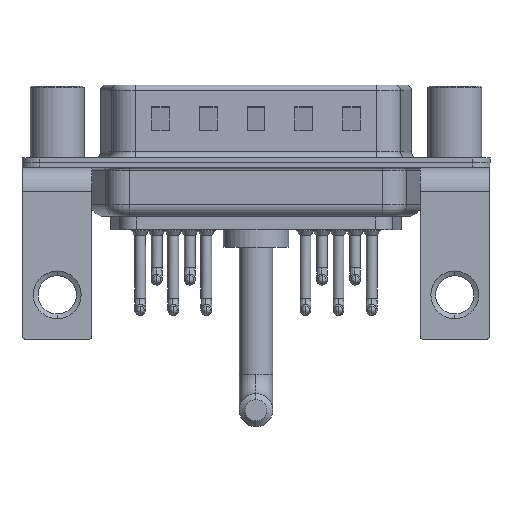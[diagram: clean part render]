
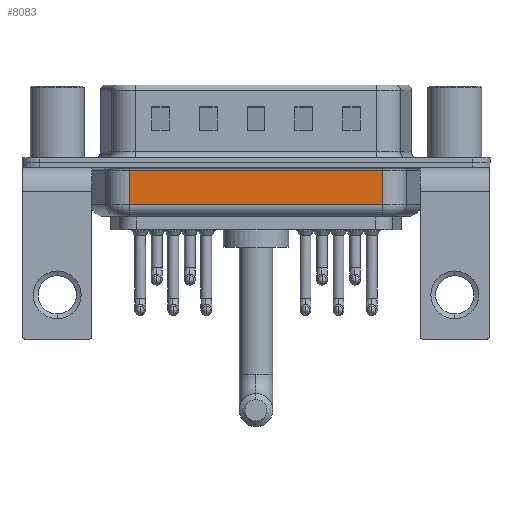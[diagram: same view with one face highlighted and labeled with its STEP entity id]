
A CAD part, front view. The second image highlights one B-rep face of the part: STEP entity #8083.
In plain terms, the highlighted planar face has unit normal (0, -1, 0).
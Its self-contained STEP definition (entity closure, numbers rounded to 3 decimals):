
#132 = CARTESIAN_POINT ( 'NONE',  ( 27.269, -5.35, -0.65 ) ) ;
#487 = CARTESIAN_POINT ( 'NONE',  ( 6.031, -5.35, -0.65 ) ) ;
#1815 = ORIENTED_EDGE ( 'NONE', *, *, #18002, .T. ) ;
#2347 = VECTOR ( 'NONE', #18919, 1000. ) ;
#2544 = FACE_OUTER_BOUND ( 'NONE', #10733, .T. ) ;
#3150 = DIRECTION ( 'NONE',  ( 0., 0., 1. ) ) ;
#3203 = VERTEX_POINT ( 'NONE', #10201 ) ;
#3231 = EDGE_CURVE ( 'NONE', #3203, #4375, #22503, .T. ) ;
#3265 = LINE ( 'NONE', #9213, #8593 ) ;
#4199 = PLANE ( 'NONE',  #16189 ) ;
#4375 = VERTEX_POINT ( 'NONE', #132 ) ;
#4764 = ORIENTED_EDGE ( 'NONE', *, *, #3231, .T. ) ;
#7668 = EDGE_CURVE ( 'NONE', #4375, #11059, #18162, .T. ) ;
#8083 = ADVANCED_FACE ( 'NONE', ( #2544 ), #4199, .F. ) ;
#8593 = VECTOR ( 'NONE', #3150, 1000. ) ;
#9213 = CARTESIAN_POINT ( 'NONE',  ( 6.031, -5.35, -4.5 ) ) ;
#9237 = VECTOR ( 'NONE', #12016, 1000. ) ;
#9753 = ORIENTED_EDGE ( 'NONE', *, *, #7668, .T. ) ;
#10102 = CARTESIAN_POINT ( 'NONE',  ( 6.031, -5.35, -4.5 ) ) ;
#10201 = CARTESIAN_POINT ( 'NONE',  ( 27.269, -5.35, -3.5 ) ) ;
#10733 = EDGE_LOOP ( 'NONE', ( #10746, #1815, #4764, #9753 ) ) ;
#10746 = ORIENTED_EDGE ( 'NONE', *, *, #24765, .F. ) ;
#11059 = VERTEX_POINT ( 'NONE', #487 ) ;
#11062 = CARTESIAN_POINT ( 'NONE',  ( 27.269, -5.35, -4.5 ) ) ;
#11434 = VERTEX_POINT ( 'NONE', #13946 ) ;
#11792 = VECTOR ( 'NONE', #14943, 1000. ) ;
#12016 = DIRECTION ( 'NONE',  ( -1., 0., 0. ) ) ;
#13946 = CARTESIAN_POINT ( 'NONE',  ( 6.031, -5.35, -3.5 ) ) ;
#14943 = DIRECTION ( 'NONE',  ( 0., 0., 1. ) ) ;
#16189 = AXIS2_PLACEMENT_3D ( 'NONE', #10102, #19538, #23687 ) ;
#18002 = EDGE_CURVE ( 'NONE', #11434, #3203, #24237, .T. ) ;
#18162 = LINE ( 'NONE', #20053, #9237 ) ;
#18919 = DIRECTION ( 'NONE',  ( 1., 0., 0. ) ) ;
#19538 = DIRECTION ( 'NONE',  ( 0., 1., 0. ) ) ;
#20053 = CARTESIAN_POINT ( 'NONE',  ( 6.031, -5.35, -0.65 ) ) ;
#22503 = LINE ( 'NONE', #11062, #11792 ) ;
#23687 = DIRECTION ( 'NONE',  ( 0., 0., 1. ) ) ;
#24237 = LINE ( 'NONE', #24361, #2347 ) ;
#24361 = CARTESIAN_POINT ( 'NONE',  ( 6.031, -5.35, -3.5 ) ) ;
#24765 = EDGE_CURVE ( 'NONE', #11434, #11059, #3265, .T. ) ;
